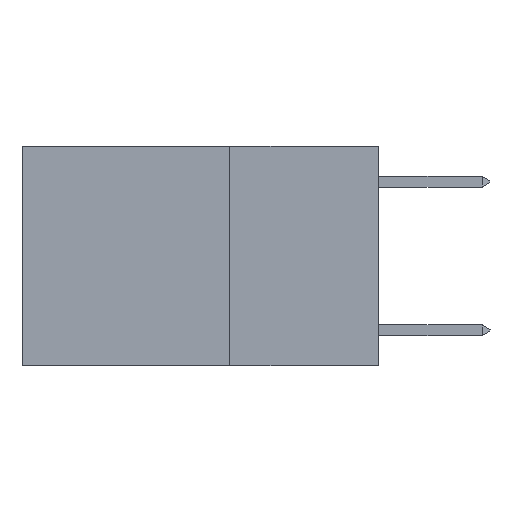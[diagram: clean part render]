
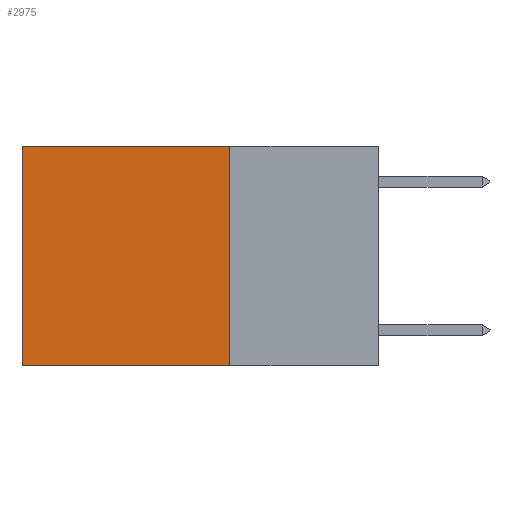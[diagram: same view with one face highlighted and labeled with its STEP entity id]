
A CAD part, left-side view. The second image highlights one B-rep face of the part: STEP entity #2975.
In plain terms, the highlighted planar face has unit normal (-1, 0, 0).
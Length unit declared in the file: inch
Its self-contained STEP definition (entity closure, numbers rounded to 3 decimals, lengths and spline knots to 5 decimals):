
#47 = LINE ( 'NONE', #10903, #7128 ) ;
#279 = VERTEX_POINT ( 'NONE', #3701 ) ;
#1545 = VECTOR ( 'NONE', #13628, 39.37008 ) ;
#1712 = DIRECTION ( 'NONE',  ( 0., 1., 0. ) ) ;
#1904 = PLANE ( 'NONE',  #3550 ) ;
#2941 = CARTESIAN_POINT ( 'NONE',  ( 0.2625, 0.25, -0.37 ) ) ;
#2975 = ADVANCED_FACE ( 'NONE', ( #13820 ), #1904, .F. ) ;
#3246 = EDGE_CURVE ( 'NONE', #279, #16210, #47, .T. ) ;
#3331 = ORIENTED_EDGE ( 'NONE', *, *, #3246, .T. ) ;
#3550 = AXIS2_PLACEMENT_3D ( 'NONE', #5931, #13040, #10481 ) ;
#3701 = CARTESIAN_POINT ( 'NONE',  ( 0.2625, 0.6, 0. ) ) ;
#4077 = CARTESIAN_POINT ( 'NONE',  ( 0.2625, 0.25, 0. ) ) ;
#4250 = LINE ( 'NONE', #4077, #13039 ) ;
#4332 = LINE ( 'NONE', #2941, #1545 ) ;
#4922 = LINE ( 'NONE', #15626, #4980 ) ;
#4980 = VECTOR ( 'NONE', #15534, 39.37008 ) ;
#5931 = CARTESIAN_POINT ( 'NONE',  ( 0.2625, 0.25, 0. ) ) ;
#6207 = EDGE_CURVE ( 'NONE', #6827, #279, #4250, .T. ) ;
#6827 = VERTEX_POINT ( 'NONE', #14109 ) ;
#6842 = DIRECTION ( 'NONE',  ( 0., 0., -1. ) ) ;
#7128 = VECTOR ( 'NONE', #6842, 39.37008 ) ;
#7277 = CARTESIAN_POINT ( 'NONE',  ( 0.2625, 0.25, -0.37 ) ) ;
#7527 = EDGE_CURVE ( 'NONE', #17089, #16210, #4332, .T. ) ;
#10481 = DIRECTION ( 'NONE',  ( 0., 0., -1. ) ) ;
#10616 = ORIENTED_EDGE ( 'NONE', *, *, #6207, .T. ) ;
#10903 = CARTESIAN_POINT ( 'NONE',  ( 0.2625, 0.6, 0. ) ) ;
#11834 = ORIENTED_EDGE ( 'NONE', *, *, #7527, .F. ) ;
#13039 = VECTOR ( 'NONE', #1712, 39.37008 ) ;
#13040 = DIRECTION ( 'NONE',  ( 1., 0., 0. ) ) ;
#13500 = ORIENTED_EDGE ( 'NONE', *, *, #16435, .F. ) ;
#13628 = DIRECTION ( 'NONE',  ( 0., 1., 0. ) ) ;
#13820 = FACE_OUTER_BOUND ( 'NONE', #17073, .T. ) ;
#14109 = CARTESIAN_POINT ( 'NONE',  ( 0.2625, 0.25, 0. ) ) ;
#15534 = DIRECTION ( 'NONE',  ( 0., 0., -1. ) ) ;
#15626 = CARTESIAN_POINT ( 'NONE',  ( 0.2625, 0.25, 0. ) ) ;
#16210 = VERTEX_POINT ( 'NONE', #16558 ) ;
#16435 = EDGE_CURVE ( 'NONE', #6827, #17089, #4922, .T. ) ;
#16558 = CARTESIAN_POINT ( 'NONE',  ( 0.2625, 0.6, -0.37 ) ) ;
#17073 = EDGE_LOOP ( 'NONE', ( #3331, #11834, #13500, #10616 ) ) ;
#17089 = VERTEX_POINT ( 'NONE', #7277 ) ;
